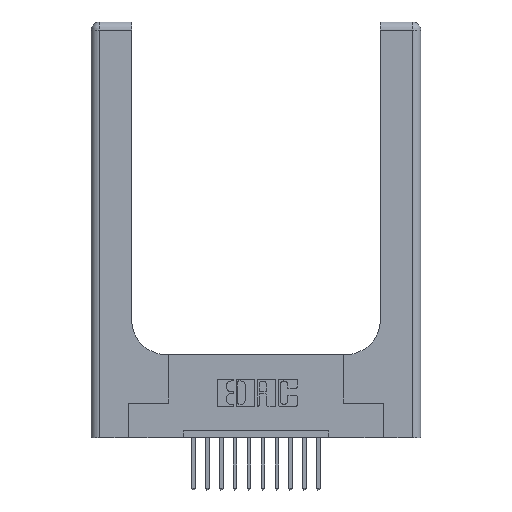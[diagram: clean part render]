
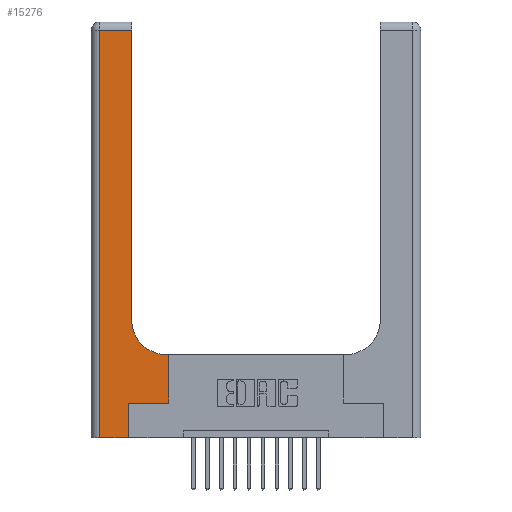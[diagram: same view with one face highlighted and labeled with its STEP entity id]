
A CAD part, top view. The second image highlights one B-rep face of the part: STEP entity #15276.
In plain terms, the highlighted planar face has unit normal (0, 0, 1).
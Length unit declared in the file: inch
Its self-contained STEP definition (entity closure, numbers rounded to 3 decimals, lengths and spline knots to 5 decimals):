
#15 = CARTESIAN_POINT ( 'NONE',  ( 0.06, 2.94, 0.37 ) ) ;
#63 = PLANE ( 'NONE',  #2358 ) ;
#157 = CARTESIAN_POINT ( 'NONE',  ( 0.06, 0., 0.37 ) ) ;
#222 = LINE ( 'NONE', #963, #1470 ) ;
#383 = ORIENTED_EDGE ( 'NONE', *, *, #10583, .T. ) ;
#484 = CARTESIAN_POINT ( 'NONE',  ( 0.2915, 0.85, 0.37 ) ) ;
#575 = ORIENTED_EDGE ( 'NONE', *, *, #7040, .T. ) ;
#671 = ORIENTED_EDGE ( 'NONE', *, *, #10845, .T. ) ;
#708 = EDGE_LOOP ( 'NONE', ( #15831, #575, #671, #16947, #8475, #2057, #11030, #383, #5755 ) ) ;
#963 = CARTESIAN_POINT ( 'NONE',  ( 0.2915, 3., 0.37 ) ) ;
#1210 = VECTOR ( 'NONE', #2425, 39.37008 ) ;
#1470 = VECTOR ( 'NONE', #6915, 39.37008 ) ;
#1651 = CARTESIAN_POINT ( 'NONE',  ( 0.269, 0.25, 0.37 ) ) ;
#1725 = DIRECTION ( 'NONE',  ( 1., 0., 0. ) ) ;
#2025 = VECTOR ( 'NONE', #4203, 39.37008 ) ;
#2057 = ORIENTED_EDGE ( 'NONE', *, *, #12795, .T. ) ;
#2358 = AXIS2_PLACEMENT_3D ( 'NONE', #13040, #2578, #3934 ) ;
#2425 = DIRECTION ( 'NONE',  ( -1., 0., 0. ) ) ;
#2578 = DIRECTION ( 'NONE',  ( 0., 0., -1. ) ) ;
#2778 = VERTEX_POINT ( 'NONE', #1651 ) ;
#2879 = FACE_OUTER_BOUND ( 'NONE', #708, .T. ) ;
#2908 = CARTESIAN_POINT ( 'NONE',  ( 0.5585, 0.25, 0.37 ) ) ;
#3505 = CARTESIAN_POINT ( 'NONE',  ( 0.06, 3., 0.37 ) ) ;
#3638 = CARTESIAN_POINT ( 'NONE',  ( 0.269, 0., 0.37 ) ) ;
#3783 = CARTESIAN_POINT ( 'NONE',  ( 0., 2.94, 0.37 ) ) ;
#3932 = DIRECTION ( 'NONE',  ( 0., 1., 0. ) ) ;
#3934 = DIRECTION ( 'NONE',  ( -1., 0., 0. ) ) ;
#4203 = DIRECTION ( 'NONE',  ( -1., 0., 0. ) ) ;
#4208 = CARTESIAN_POINT ( 'NONE',  ( 0., 0., 0.37 ) ) ;
#4423 = CARTESIAN_POINT ( 'NONE',  ( 0.2915, 2.94, 0.37 ) ) ;
#4436 = CARTESIAN_POINT ( 'NONE',  ( 0.5415, 0.85, 0.37 ) ) ;
#4696 = LINE ( 'NONE', #3638, #10261 ) ;
#4723 = DIRECTION ( 'NONE',  ( 1., 0., 0. ) ) ;
#4890 = EDGE_CURVE ( 'NONE', #13612, #6469, #12406, .T. ) ;
#5359 = VERTEX_POINT ( 'NONE', #15 ) ;
#5379 = EDGE_CURVE ( 'NONE', #6469, #10250, #222, .T. ) ;
#5694 = VERTEX_POINT ( 'NONE', #12603 ) ;
#5755 = ORIENTED_EDGE ( 'NONE', *, *, #4890, .T. ) ;
#6033 = CARTESIAN_POINT ( 'NONE',  ( 0.5585, 0.6, 0.37 ) ) ;
#6325 = VERTEX_POINT ( 'NONE', #6033 ) ;
#6469 = VERTEX_POINT ( 'NONE', #484 ) ;
#6915 = DIRECTION ( 'NONE',  ( 0., 1., 0. ) ) ;
#6983 = VECTOR ( 'NONE', #13412, 39.37008 ) ;
#7040 = EDGE_CURVE ( 'NONE', #10250, #5359, #14619, .T. ) ;
#7330 = VERTEX_POINT ( 'NONE', #2908 ) ;
#7398 = DIRECTION ( 'NONE',  ( 0., -1., 0. ) ) ;
#7871 = EDGE_CURVE ( 'NONE', #16182, #5694, #10861, .T. ) ;
#8475 = ORIENTED_EDGE ( 'NONE', *, *, #10360, .T. ) ;
#9127 = LINE ( 'NONE', #11995, #15310 ) ;
#9744 = DIRECTION ( 'NONE',  ( 0., 0., -1. ) ) ;
#10250 = VERTEX_POINT ( 'NONE', #4423 ) ;
#10261 = VECTOR ( 'NONE', #16735, 39.37008 ) ;
#10360 = EDGE_CURVE ( 'NONE', #5694, #2778, #4696, .T. ) ;
#10438 = LINE ( 'NONE', #12137, #2025 ) ;
#10583 = EDGE_CURVE ( 'NONE', #6325, #13612, #10438, .T. ) ;
#10652 = LINE ( 'NONE', #3505, #10852 ) ;
#10845 = EDGE_CURVE ( 'NONE', #5359, #16182, #10652, .T. ) ;
#10852 = VECTOR ( 'NONE', #7398, 39.37008 ) ;
#10861 = LINE ( 'NONE', #4208, #6983 ) ;
#11030 = ORIENTED_EDGE ( 'NONE', *, *, #13777, .T. ) ;
#11995 = CARTESIAN_POINT ( 'NONE',  ( 0.5585, 0.25, 0.37 ) ) ;
#12137 = CARTESIAN_POINT ( 'NONE',  ( 0.2915, 0.6, 0.37 ) ) ;
#12406 = CIRCLE ( 'NONE', #16118, 0.25 ) ;
#12603 = CARTESIAN_POINT ( 'NONE',  ( 0.269, 0., 0.37 ) ) ;
#12795 = EDGE_CURVE ( 'NONE', #2778, #7330, #13705, .T. ) ;
#13040 = CARTESIAN_POINT ( 'NONE',  ( 0., 3., 0.37 ) ) ;
#13412 = DIRECTION ( 'NONE',  ( 1., 0., 0. ) ) ;
#13612 = VERTEX_POINT ( 'NONE', #16708 ) ;
#13705 = LINE ( 'NONE', #14059, #14315 ) ;
#13777 = EDGE_CURVE ( 'NONE', #7330, #6325, #9127, .T. ) ;
#14059 = CARTESIAN_POINT ( 'NONE',  ( 0.269, 0.25, 0.37 ) ) ;
#14315 = VECTOR ( 'NONE', #4723, 39.37008 ) ;
#14619 = LINE ( 'NONE', #3783, #1210 ) ;
#15276 = ADVANCED_FACE ( 'NONE', ( #2879 ), #63, .F. ) ;
#15310 = VECTOR ( 'NONE', #3932, 39.37008 ) ;
#15831 = ORIENTED_EDGE ( 'NONE', *, *, #5379, .T. ) ;
#16118 = AXIS2_PLACEMENT_3D ( 'NONE', #4436, #9744, #1725 ) ;
#16182 = VERTEX_POINT ( 'NONE', #157 ) ;
#16708 = CARTESIAN_POINT ( 'NONE',  ( 0.5415, 0.6, 0.37 ) ) ;
#16735 = DIRECTION ( 'NONE',  ( 0., 1., 0. ) ) ;
#16947 = ORIENTED_EDGE ( 'NONE', *, *, #7871, .T. ) ;
